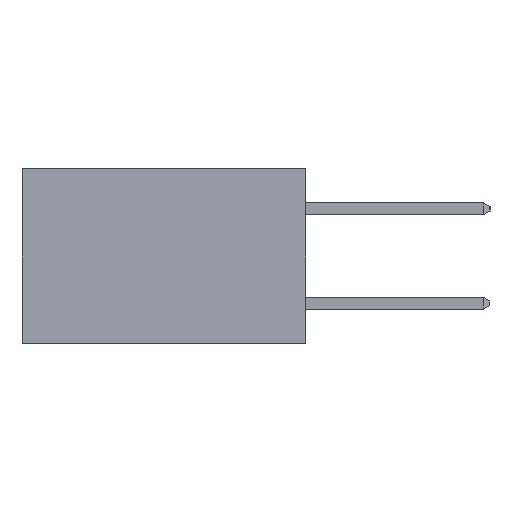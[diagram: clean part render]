
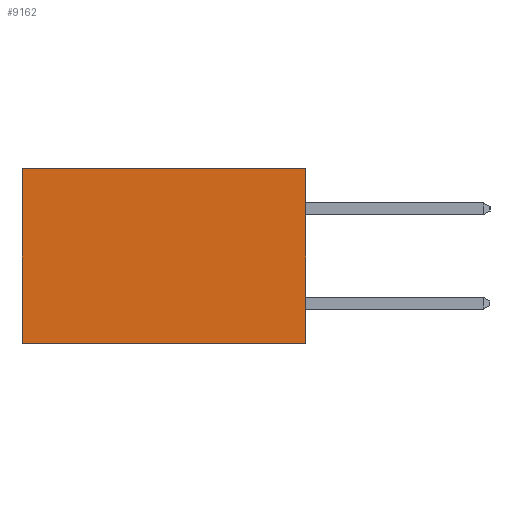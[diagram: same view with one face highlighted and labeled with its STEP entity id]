
A CAD part, left-side view. The second image highlights one B-rep face of the part: STEP entity #9162.
In plain terms, the highlighted planar face has unit normal (-1, 0, 0).
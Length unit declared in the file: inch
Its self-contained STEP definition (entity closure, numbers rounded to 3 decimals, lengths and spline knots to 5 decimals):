
#454 = PLANE ( 'NONE',  #25281 ) ;
#598 = LINE ( 'NONE', #8891, #19463 ) ;
#1234 = LINE ( 'NONE', #1360, #18738 ) ;
#1360 = CARTESIAN_POINT ( 'NONE',  ( 0.2615, 0.6, -0.37 ) ) ;
#1933 = ORIENTED_EDGE ( 'NONE', *, *, #4035, .F. ) ;
#2489 = CARTESIAN_POINT ( 'NONE',  ( 0.2615, 0., -0.37 ) ) ;
#3233 = LINE ( 'NONE', #8955, #21967 ) ;
#4035 = EDGE_CURVE ( 'NONE', #14450, #21831, #3233, .T. ) ;
#5118 = ORIENTED_EDGE ( 'NONE', *, *, #20654, .F. ) ;
#5699 = LINE ( 'NONE', #9914, #15937 ) ;
#6927 = CARTESIAN_POINT ( 'NONE',  ( 0.2615, 0., 0. ) ) ;
#8741 = DIRECTION ( 'NONE',  ( 0., 0., -1. ) ) ;
#8891 = CARTESIAN_POINT ( 'NONE',  ( 0.2615, 0., 0. ) ) ;
#8955 = CARTESIAN_POINT ( 'NONE',  ( 0.2615, 0., -0.37 ) ) ;
#9162 = ADVANCED_FACE ( 'NONE', ( #14723 ), #454, .F. ) ;
#9914 = CARTESIAN_POINT ( 'NONE',  ( 0.2615, 0., -0.37 ) ) ;
#10129 = CARTESIAN_POINT ( 'NONE',  ( 0.2615, 0., -0.37 ) ) ;
#10769 = CARTESIAN_POINT ( 'NONE',  ( 0.2615, 0.6, -0.37 ) ) ;
#11104 = EDGE_LOOP ( 'NONE', ( #24746, #1933, #5118, #23152 ) ) ;
#11569 = VERTEX_POINT ( 'NONE', #16507 ) ;
#11775 = EDGE_CURVE ( 'NONE', #11569, #21831, #1234, .T. ) ;
#14450 = VERTEX_POINT ( 'NONE', #10129 ) ;
#14723 = FACE_OUTER_BOUND ( 'NONE', #11104, .T. ) ;
#14840 = DIRECTION ( 'NONE',  ( 1., 0., 0. ) ) ;
#15937 = VECTOR ( 'NONE', #18182, 39.37008 ) ;
#16507 = CARTESIAN_POINT ( 'NONE',  ( 0.2615, 0.6, 0. ) ) ;
#17228 = DIRECTION ( 'NONE',  ( 0., 1., 0. ) ) ;
#17426 = DIRECTION ( 'NONE',  ( 0., 1., 0. ) ) ;
#18182 = DIRECTION ( 'NONE',  ( 0., 0., -1. ) ) ;
#18738 = VECTOR ( 'NONE', #24166, 39.37008 ) ;
#19463 = VECTOR ( 'NONE', #17426, 39.37008 ) ;
#20654 = EDGE_CURVE ( 'NONE', #24640, #14450, #5699, .T. ) ;
#21831 = VERTEX_POINT ( 'NONE', #10769 ) ;
#21967 = VECTOR ( 'NONE', #17228, 39.37008 ) ;
#23152 = ORIENTED_EDGE ( 'NONE', *, *, #24005, .T. ) ;
#24005 = EDGE_CURVE ( 'NONE', #24640, #11569, #598, .T. ) ;
#24166 = DIRECTION ( 'NONE',  ( 0., 0., -1. ) ) ;
#24640 = VERTEX_POINT ( 'NONE', #6927 ) ;
#24746 = ORIENTED_EDGE ( 'NONE', *, *, #11775, .T. ) ;
#25281 = AXIS2_PLACEMENT_3D ( 'NONE', #2489, #14840, #8741 ) ;
